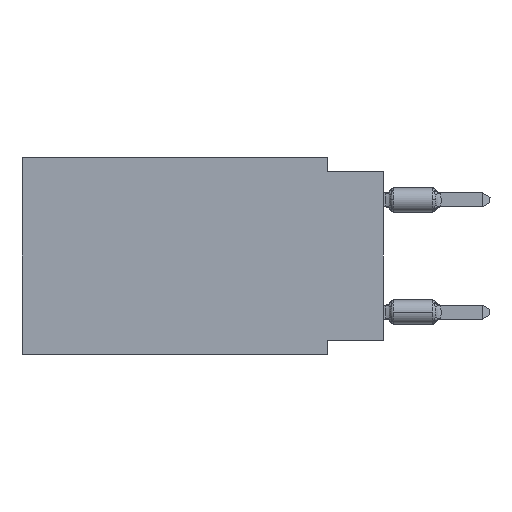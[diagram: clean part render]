
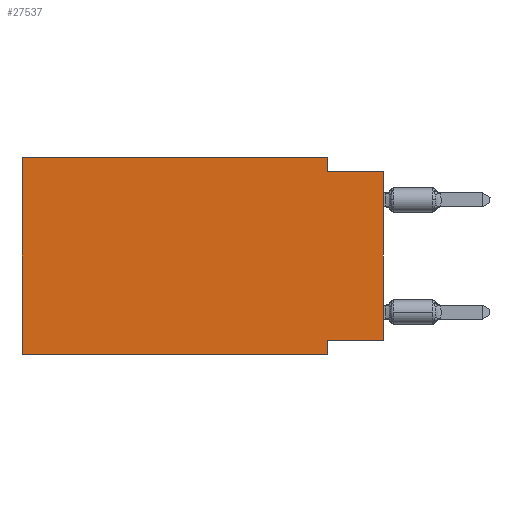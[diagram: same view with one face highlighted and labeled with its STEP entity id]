
A CAD part, left-side view. The second image highlights one B-rep face of the part: STEP entity #27537.
In plain terms, the highlighted planar face has unit normal (-1, 0, 0).
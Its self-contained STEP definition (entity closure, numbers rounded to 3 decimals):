
#103 = LINE ( 'NONE', #19382, #20303 ) ;
#1095 = VECTOR ( 'NONE', #12407, 1000. ) ;
#1398 = VECTOR ( 'NONE', #26825, 1000. ) ;
#1515 = CARTESIAN_POINT ( 'NONE',  ( 0., 16.383, -8.89 ) ) ;
#1693 = ORIENTED_EDGE ( 'NONE', *, *, #9898, .F. ) ;
#1988 = ORIENTED_EDGE ( 'NONE', *, *, #9035, .T. ) ;
#2572 = DIRECTION ( 'NONE',  ( 0., 0., -1. ) ) ;
#3487 = VERTEX_POINT ( 'NONE', #10110 ) ;
#3674 = LINE ( 'NONE', #26823, #22054 ) ;
#4347 = FACE_OUTER_BOUND ( 'NONE', #5546, .T. ) ;
#5546 = EDGE_LOOP ( 'NONE', ( #9052, #18471, #23861, #18367, #8201, #1988, #18379, #1693 ) ) ;
#5845 = EDGE_CURVE ( 'NONE', #26368, #24734, #11947, .T. ) ;
#6049 = CARTESIAN_POINT ( 'NONE',  ( 0., 0., -8.255 ) ) ;
#6256 = EDGE_CURVE ( 'NONE', #6259, #10431, #19013, .T. ) ;
#6259 = VERTEX_POINT ( 'NONE', #28592 ) ;
#6592 = LINE ( 'NONE', #21094, #21088 ) ;
#6758 = VECTOR ( 'NONE', #22713, 1000. ) ;
#7856 = DIRECTION ( 'NONE',  ( 0., 0., -1. ) ) ;
#7893 = VERTEX_POINT ( 'NONE', #14494 ) ;
#8201 = ORIENTED_EDGE ( 'NONE', *, *, #10846, .F. ) ;
#9035 = EDGE_CURVE ( 'NONE', #3487, #12984, #27439, .T. ) ;
#9052 = ORIENTED_EDGE ( 'NONE', *, *, #6256, .T. ) ;
#9898 = EDGE_CURVE ( 'NONE', #6259, #24424, #20701, .T. ) ;
#10110 = CARTESIAN_POINT ( 'NONE',  ( 0., 16.383, -8.89 ) ) ;
#10431 = VERTEX_POINT ( 'NONE', #26030 ) ;
#10846 = EDGE_CURVE ( 'NONE', #3487, #26368, #6592, .T. ) ;
#11144 = CARTESIAN_POINT ( 'NONE',  ( 0., 2.54, 0. ) ) ;
#11759 = CARTESIAN_POINT ( 'NONE',  ( 0., 2.54, -8.89 ) ) ;
#11947 = LINE ( 'NONE', #18752, #1095 ) ;
#12407 = DIRECTION ( 'NONE',  ( 0., -1., 0. ) ) ;
#12984 = VERTEX_POINT ( 'NONE', #11759 ) ;
#13124 = VECTOR ( 'NONE', #22493, 1000. ) ;
#14494 = CARTESIAN_POINT ( 'NONE',  ( 0., 2.54, -0.635 ) ) ;
#16011 = AXIS2_PLACEMENT_3D ( 'NONE', #23467, #23628, #18700 ) ;
#16487 = VECTOR ( 'NONE', #28088, 1000. ) ;
#16819 = EDGE_CURVE ( 'NONE', #24734, #7893, #103, .T. ) ;
#18367 = ORIENTED_EDGE ( 'NONE', *, *, #5845, .F. ) ;
#18379 = ORIENTED_EDGE ( 'NONE', *, *, #25308, .F. ) ;
#18471 = ORIENTED_EDGE ( 'NONE', *, *, #20355, .F. ) ;
#18673 = CARTESIAN_POINT ( 'NONE',  ( 0., 0., -0.635 ) ) ;
#18700 = DIRECTION ( 'NONE',  ( 0., 0., -1. ) ) ;
#18752 = CARTESIAN_POINT ( 'NONE',  ( 0., 16.383, 0. ) ) ;
#18848 = PLANE ( 'NONE',  #16011 ) ;
#18934 = DIRECTION ( 'NONE',  ( 0., 0., 1. ) ) ;
#19013 = LINE ( 'NONE', #23326, #1398 ) ;
#19054 = CARTESIAN_POINT ( 'NONE',  ( 0., 2.54, -8.255 ) ) ;
#19382 = CARTESIAN_POINT ( 'NONE',  ( 0., 2.54, 0. ) ) ;
#20303 = VECTOR ( 'NONE', #2572, 1000. ) ;
#20355 = EDGE_CURVE ( 'NONE', #7893, #10431, #21123, .T. ) ;
#20701 = LINE ( 'NONE', #6049, #6758 ) ;
#21088 = VECTOR ( 'NONE', #18934, 1000. ) ;
#21094 = CARTESIAN_POINT ( 'NONE',  ( 0., 16.383, 0. ) ) ;
#21123 = LINE ( 'NONE', #18673, #16487 ) ;
#22054 = VECTOR ( 'NONE', #7856, 1000. ) ;
#22493 = DIRECTION ( 'NONE',  ( 0., -1., 0. ) ) ;
#22713 = DIRECTION ( 'NONE',  ( 0., 1., 0. ) ) ;
#23326 = CARTESIAN_POINT ( 'NONE',  ( 0., 0., 0. ) ) ;
#23467 = CARTESIAN_POINT ( 'NONE',  ( 0., 16.383, 0. ) ) ;
#23628 = DIRECTION ( 'NONE',  ( 1., 0., 0. ) ) ;
#23861 = ORIENTED_EDGE ( 'NONE', *, *, #16819, .F. ) ;
#24424 = VERTEX_POINT ( 'NONE', #19054 ) ;
#24734 = VERTEX_POINT ( 'NONE', #11144 ) ;
#25308 = EDGE_CURVE ( 'NONE', #24424, #12984, #3674, .T. ) ;
#26030 = CARTESIAN_POINT ( 'NONE',  ( 0., 0., -0.635 ) ) ;
#26368 = VERTEX_POINT ( 'NONE', #28368 ) ;
#26823 = CARTESIAN_POINT ( 'NONE',  ( 0., 2.54, -8.89 ) ) ;
#26825 = DIRECTION ( 'NONE',  ( 0., 0., 1. ) ) ;
#27439 = LINE ( 'NONE', #1515, #13124 ) ;
#27537 = ADVANCED_FACE ( 'NONE', ( #4347 ), #18848, .F. ) ;
#28088 = DIRECTION ( 'NONE',  ( 0., -1., 0. ) ) ;
#28368 = CARTESIAN_POINT ( 'NONE',  ( 0., 16.383, 0. ) ) ;
#28592 = CARTESIAN_POINT ( 'NONE',  ( 0., 0., -8.255 ) ) ;
